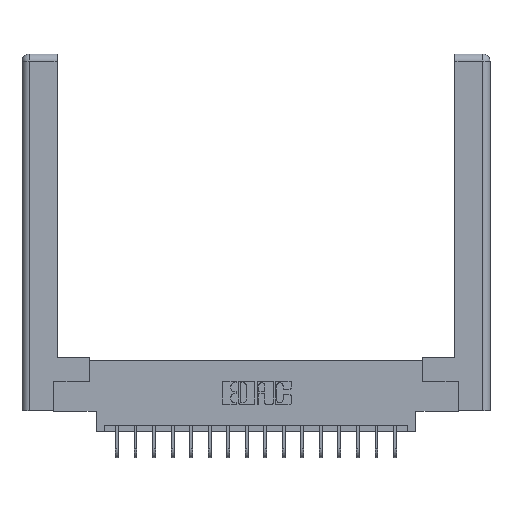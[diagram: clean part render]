
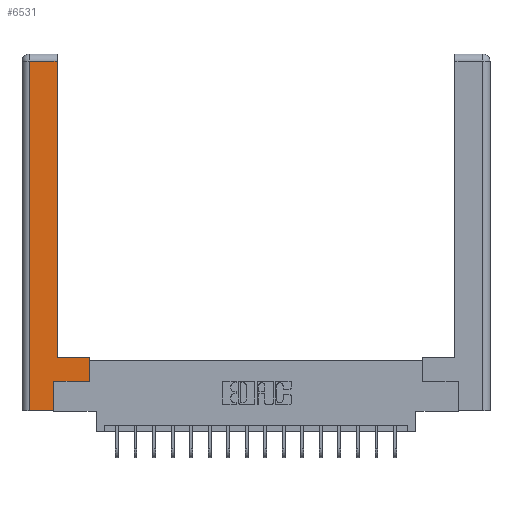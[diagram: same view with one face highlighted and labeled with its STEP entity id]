
A CAD part, top view. The second image highlights one B-rep face of the part: STEP entity #6531.
In plain terms, the highlighted planar face has unit normal (0, 0, 1).
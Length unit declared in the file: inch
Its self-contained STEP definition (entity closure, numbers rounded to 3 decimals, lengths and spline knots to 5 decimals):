
#290 = CARTESIAN_POINT ( 'NONE',  ( 0.0615, 2.94, 0. ) ) ;
#1156 = CARTESIAN_POINT ( 'NONE',  ( 0., 0., 0. ) ) ;
#1184 = DIRECTION ( 'NONE',  ( 0., 1., 0. ) ) ;
#1221 = VECTOR ( 'NONE', #18184, 39.37008 ) ;
#1343 = VECTOR ( 'NONE', #12909, 39.37008 ) ;
#1527 = ORIENTED_EDGE ( 'NONE', *, *, #17850, .T. ) ;
#1690 = LINE ( 'NONE', #20347, #16676 ) ;
#2017 = VECTOR ( 'NONE', #15883, 39.37008 ) ;
#2301 = ORIENTED_EDGE ( 'NONE', *, *, #4209, .T. ) ;
#2501 = LINE ( 'NONE', #8175, #2017 ) ;
#3450 = CARTESIAN_POINT ( 'NONE',  ( 0.565, 0.245, 0. ) ) ;
#4109 = CARTESIAN_POINT ( 'NONE',  ( 0.565, 0.45, 0. ) ) ;
#4209 = EDGE_CURVE ( 'NONE', #15793, #19714, #8621, .T. ) ;
#4944 = CARTESIAN_POINT ( 'NONE',  ( 0.295, 3., 0. ) ) ;
#5065 = EDGE_CURVE ( 'NONE', #9187, #9816, #6616, .T. ) ;
#5643 = CARTESIAN_POINT ( 'NONE',  ( 0.0615, 0., 0. ) ) ;
#5849 = DIRECTION ( 'NONE',  ( 1., 0., 0. ) ) ;
#6037 = DIRECTION ( 'NONE',  ( -1., 0., 0. ) ) ;
#6163 = EDGE_LOOP ( 'NONE', ( #2301, #1527, #10012, #7480, #14626, #6963, #16632, #20114 ) ) ;
#6208 = EDGE_CURVE ( 'NONE', #7017, #10686, #2501, .T. ) ;
#6531 = ADVANCED_FACE ( 'NONE', ( #19188 ), #18509, .F. ) ;
#6616 = LINE ( 'NONE', #5643, #1221 ) ;
#6963 = ORIENTED_EDGE ( 'NONE', *, *, #19260, .T. ) ;
#7017 = VERTEX_POINT ( 'NONE', #13513 ) ;
#7480 = ORIENTED_EDGE ( 'NONE', *, *, #17655, .T. ) ;
#7563 = CARTESIAN_POINT ( 'NONE',  ( 0.295, 2.94, 0. ) ) ;
#8175 = CARTESIAN_POINT ( 'NONE',  ( 0.265, 0.245, 0. ) ) ;
#8621 = LINE ( 'NONE', #4944, #10337 ) ;
#8843 = EDGE_CURVE ( 'NONE', #9838, #15793, #1690, .T. ) ;
#8939 = CARTESIAN_POINT ( 'NONE',  ( 0.265, 0., 0. ) ) ;
#9024 = CARTESIAN_POINT ( 'NONE',  ( 0.265, 0.245, 0. ) ) ;
#9187 = VERTEX_POINT ( 'NONE', #11367 ) ;
#9270 = AXIS2_PLACEMENT_3D ( 'NONE', #1156, #15458, #6037 ) ;
#9566 = DIRECTION ( 'NONE',  ( 0., 1., 0. ) ) ;
#9694 = LINE ( 'NONE', #4109, #12929 ) ;
#9816 = VERTEX_POINT ( 'NONE', #15774 ) ;
#9838 = VERTEX_POINT ( 'NONE', #15558 ) ;
#10012 = ORIENTED_EDGE ( 'NONE', *, *, #5065, .T. ) ;
#10182 = LINE ( 'NONE', #290, #18025 ) ;
#10337 = VECTOR ( 'NONE', #9566, 39.37008 ) ;
#10686 = VERTEX_POINT ( 'NONE', #9024 ) ;
#11367 = CARTESIAN_POINT ( 'NONE',  ( 0.0615, 2.94, 0. ) ) ;
#12909 = DIRECTION ( 'NONE',  ( 1., 0., 0. ) ) ;
#12929 = VECTOR ( 'NONE', #1184, 39.37008 ) ;
#13291 = CARTESIAN_POINT ( 'NONE',  ( 0.295, 0.45, 0. ) ) ;
#13513 = CARTESIAN_POINT ( 'NONE',  ( 0.265, 0., 0. ) ) ;
#13883 = VECTOR ( 'NONE', #5849, 39.37008 ) ;
#13892 = LINE ( 'NONE', #3450, #1343 ) ;
#14255 = DIRECTION ( 'NONE',  ( -1., 0., 0. ) ) ;
#14337 = VERTEX_POINT ( 'NONE', #15294 ) ;
#14444 = DIRECTION ( 'NONE',  ( -1., 0., 0. ) ) ;
#14626 = ORIENTED_EDGE ( 'NONE', *, *, #6208, .T. ) ;
#15294 = CARTESIAN_POINT ( 'NONE',  ( 0.565, 0.245, 0. ) ) ;
#15458 = DIRECTION ( 'NONE',  ( 0., 0., -1. ) ) ;
#15558 = CARTESIAN_POINT ( 'NONE',  ( 0.565, 0.45, 0. ) ) ;
#15774 = CARTESIAN_POINT ( 'NONE',  ( 0.0615, 0., 0. ) ) ;
#15793 = VERTEX_POINT ( 'NONE', #13291 ) ;
#15883 = DIRECTION ( 'NONE',  ( 0., 1., 0. ) ) ;
#16632 = ORIENTED_EDGE ( 'NONE', *, *, #17688, .T. ) ;
#16676 = VECTOR ( 'NONE', #14255, 39.37008 ) ;
#16808 = LINE ( 'NONE', #8939, #13883 ) ;
#17655 = EDGE_CURVE ( 'NONE', #9816, #7017, #16808, .T. ) ;
#17688 = EDGE_CURVE ( 'NONE', #14337, #9838, #9694, .T. ) ;
#17850 = EDGE_CURVE ( 'NONE', #19714, #9187, #10182, .T. ) ;
#18025 = VECTOR ( 'NONE', #14444, 39.37008 ) ;
#18184 = DIRECTION ( 'NONE',  ( 0., -1., 0. ) ) ;
#18509 = PLANE ( 'NONE',  #9270 ) ;
#19188 = FACE_OUTER_BOUND ( 'NONE', #6163, .T. ) ;
#19260 = EDGE_CURVE ( 'NONE', #10686, #14337, #13892, .T. ) ;
#19714 = VERTEX_POINT ( 'NONE', #7563 ) ;
#20114 = ORIENTED_EDGE ( 'NONE', *, *, #8843, .T. ) ;
#20347 = CARTESIAN_POINT ( 'NONE',  ( 0.295, 0.45, 0. ) ) ;
